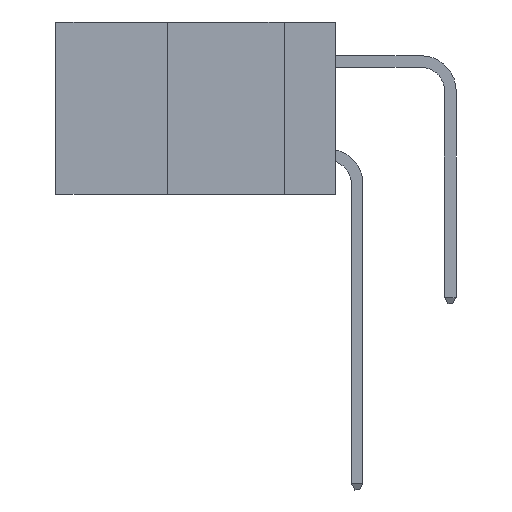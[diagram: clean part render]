
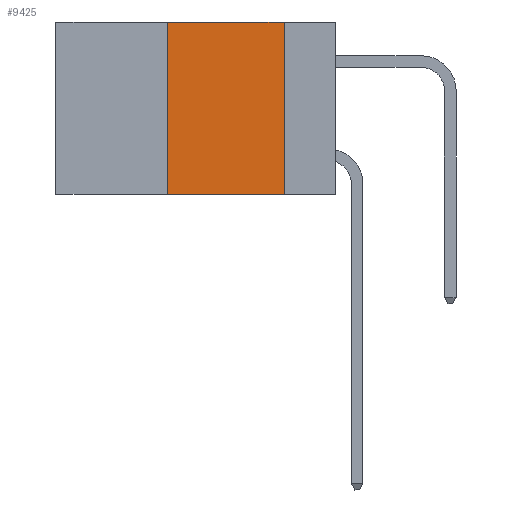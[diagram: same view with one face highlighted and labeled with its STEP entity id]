
A CAD part, left-side view. The second image highlights one B-rep face of the part: STEP entity #9425.
In plain terms, the highlighted planar face has unit normal (-1, 0, 0).
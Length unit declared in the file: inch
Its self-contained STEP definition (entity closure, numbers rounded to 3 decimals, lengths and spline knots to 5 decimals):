
#56 = VERTEX_POINT ( 'NONE', #8457 ) ;
#171 = EDGE_CURVE ( 'NONE', #2201, #56, #5735, .T. ) ;
#377 = DIRECTION ( 'NONE',  ( 0., -1., 0. ) ) ;
#515 = CARTESIAN_POINT ( 'NONE',  ( 0., 0.36, 0. ) ) ;
#611 = CARTESIAN_POINT ( 'NONE',  ( 0., 0.11, 0. ) ) ;
#1276 = EDGE_CURVE ( 'NONE', #2201, #8455, #9826, .T. ) ;
#1488 = LINE ( 'NONE', #3142, #3377 ) ;
#1592 = EDGE_CURVE ( 'NONE', #8455, #4195, #1488, .T. ) ;
#1931 = VECTOR ( 'NONE', #5178, 39.37008 ) ;
#2201 = VERTEX_POINT ( 'NONE', #5395 ) ;
#2449 = EDGE_CURVE ( 'NONE', #4195, #56, #9097, .T. ) ;
#2490 = DIRECTION ( 'NONE',  ( 0., 0., -1. ) ) ;
#3142 = CARTESIAN_POINT ( 'NONE',  ( 0., 0.6, 0. ) ) ;
#3377 = VECTOR ( 'NONE', #3827, 39.37008 ) ;
#3827 = DIRECTION ( 'NONE',  ( 0., -1., 0. ) ) ;
#4195 = VERTEX_POINT ( 'NONE', #6409 ) ;
#4427 = CARTESIAN_POINT ( 'NONE',  ( 0., 0.36, 0. ) ) ;
#4669 = ORIENTED_EDGE ( 'NONE', *, *, #2449, .F. ) ;
#4823 = FACE_OUTER_BOUND ( 'NONE', #10252, .T. ) ;
#5097 = VECTOR ( 'NONE', #2490, 39.37008 ) ;
#5178 = DIRECTION ( 'NONE',  ( 0., 0., 1. ) ) ;
#5395 = CARTESIAN_POINT ( 'NONE',  ( 0., 0.36, -0.37 ) ) ;
#5735 = LINE ( 'NONE', #5801, #8431 ) ;
#5801 = CARTESIAN_POINT ( 'NONE',  ( 0., 0.6, -0.37 ) ) ;
#5862 = CARTESIAN_POINT ( 'NONE',  ( 0., 0.6, 0. ) ) ;
#6409 = CARTESIAN_POINT ( 'NONE',  ( 0., 0.11, 0. ) ) ;
#6788 = DIRECTION ( 'NONE',  ( 1., 0., 0. ) ) ;
#6808 = AXIS2_PLACEMENT_3D ( 'NONE', #5862, #6788, #10536 ) ;
#8370 = ORIENTED_EDGE ( 'NONE', *, *, #1276, .F. ) ;
#8431 = VECTOR ( 'NONE', #377, 39.37008 ) ;
#8455 = VERTEX_POINT ( 'NONE', #4427 ) ;
#8457 = CARTESIAN_POINT ( 'NONE',  ( 0., 0.11, -0.37 ) ) ;
#8857 = ORIENTED_EDGE ( 'NONE', *, *, #171, .T. ) ;
#9097 = LINE ( 'NONE', #611, #5097 ) ;
#9425 = ADVANCED_FACE ( 'NONE', ( #4823 ), #11322, .F. ) ;
#9826 = LINE ( 'NONE', #515, #1931 ) ;
#10252 = EDGE_LOOP ( 'NONE', ( #4669, #10371, #8370, #8857 ) ) ;
#10371 = ORIENTED_EDGE ( 'NONE', *, *, #1592, .F. ) ;
#10536 = DIRECTION ( 'NONE',  ( 0., 0., -1. ) ) ;
#11322 = PLANE ( 'NONE',  #6808 ) ;
